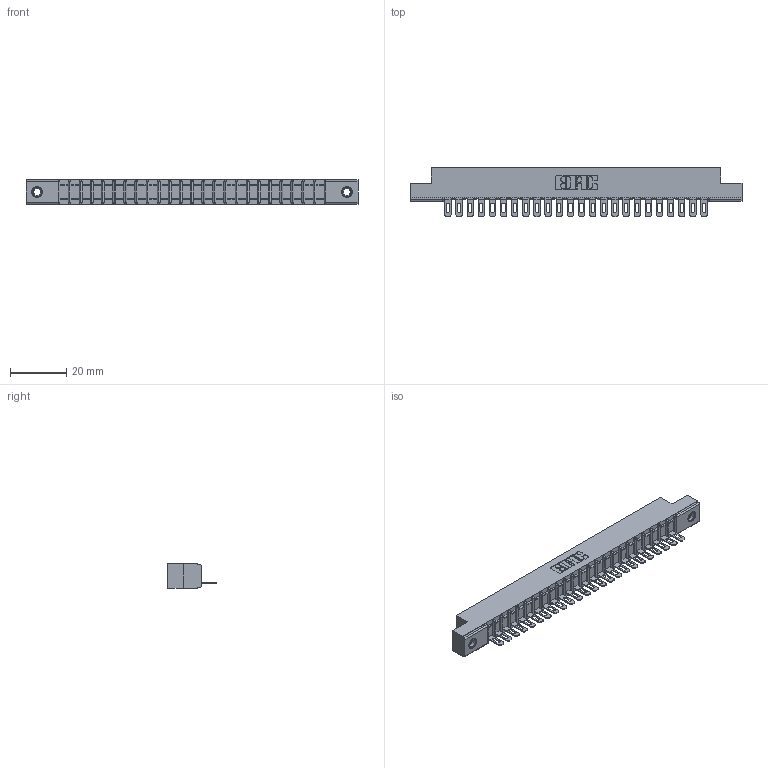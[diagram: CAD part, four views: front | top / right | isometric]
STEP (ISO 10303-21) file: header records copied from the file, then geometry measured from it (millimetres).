
FILE_DESCRIPTION (( 'STEP AP203' ), '1' );
FILE_NAME ('307-024-501-107.STEP', '2019-09-05T00:51:07', ( '' ), ( '' ), 'SwSTEP 2.0', 'SolidWorks 2016', '' );
FILE_SCHEMA (( 'CONFIG_CONTROL_DESIGN' ));
Length unit declared in the file: inch
Products named in the file (4): 345-250-001_345-250-005-103; 307 Part_.156 Dia Mounting Holes; 307-024-501-107; 307-290-002_501
Assembly tree (27 placements, depth 2):
  307-024-501-107
    307 Part_.156 Dia Mounting Holes
    307-290-002_501  x24
    345-250-001_345-250-005-103  x2
Bounding box: 118.11 x 17.42 x 8.71 mm (x, y, z)
Volume: 7805.8 mm3; surface area: 14505.8 mm2
Topology: 27 solids, 27 shells, 2027 faces, 6171 edges, 4038 vertices
Faces by surface type: plane 1158, cylinder 803, sphere 50, cone 12, torus 4
Entity records: 24773 total; most frequent: CARTESIAN_POINT 4155, ORIENTED_EDGE 4138, DIRECTION 4059, EDGE_CURVE 2069, LINE 1571, VECTOR 1571, VERTEX_POINT 1340, AXIS2_PLACEMENT_3D 1244
